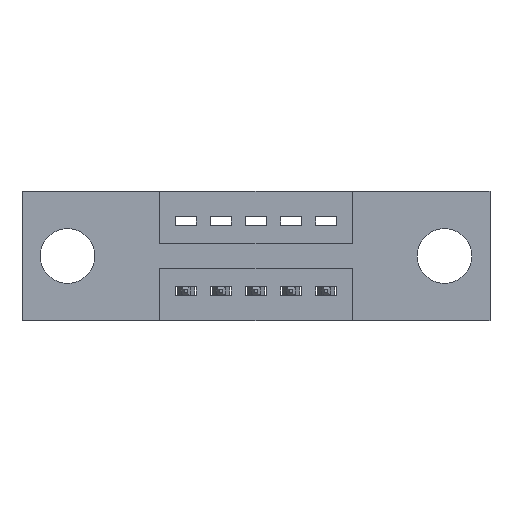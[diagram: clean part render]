
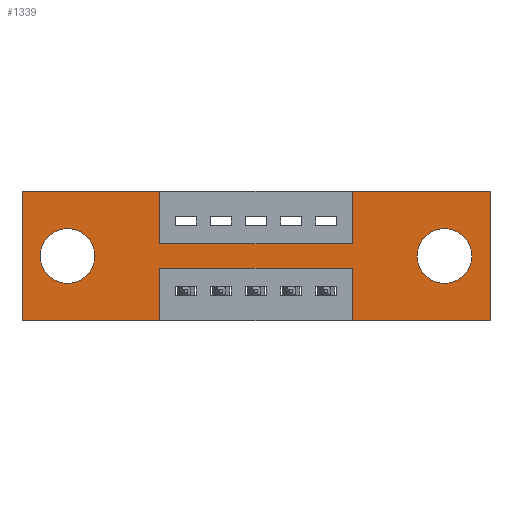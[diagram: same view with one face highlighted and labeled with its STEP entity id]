
A CAD part, front view. The second image highlights one B-rep face of the part: STEP entity #1339.
In plain terms, the highlighted planar face has unit normal (0, -1, 0).
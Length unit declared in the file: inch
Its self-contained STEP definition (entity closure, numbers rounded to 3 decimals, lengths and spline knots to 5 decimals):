
#39 = VECTOR ( 'NONE', #539, 39.37008 ) ;
#45 = VERTEX_POINT ( 'NONE', #7832 ) ;
#56 = VERTEX_POINT ( 'NONE', #8480 ) ;
#64 = CARTESIAN_POINT ( 'NONE',  ( 1.205, 0., -0.263 ) ) ;
#68 = EDGE_CURVE ( 'NONE', #2637, #4759, #3642, .T. ) ;
#254 = CARTESIAN_POINT ( 'NONE',  ( 0.3925, 0., 0. ) ) ;
#285 = LINE ( 'NONE', #3169, #6227 ) ;
#312 = CARTESIAN_POINT ( 'NONE',  ( 0.9425, 0., -0.37 ) ) ;
#321 = ORIENTED_EDGE ( 'NONE', *, *, #921, .F. ) ;
#461 = DIRECTION ( 'NONE',  ( 0., 0., -1. ) ) ;
#539 = DIRECTION ( 'NONE',  ( 0., 0., 1. ) ) ;
#630 = LINE ( 'NONE', #2152, #6124 ) ;
#632 = DIRECTION ( 'NONE',  ( 0., 0., 1. ) ) ;
#645 = VERTEX_POINT ( 'NONE', #5181 ) ;
#648 = LINE ( 'NONE', #6336, #7544 ) ;
#671 = DIRECTION ( 'NONE',  ( 1., 0., 0. ) ) ;
#755 = AXIS2_PLACEMENT_3D ( 'NONE', #7624, #4739, #4033 ) ;
#921 = EDGE_CURVE ( 'NONE', #1124, #2637, #5631, .T. ) ;
#926 = VERTEX_POINT ( 'NONE', #6422 ) ;
#1000 = CIRCLE ( 'NONE', #2480, 0.078 ) ;
#1013 = CARTESIAN_POINT ( 'NONE',  ( 0.13, 0., -0.185 ) ) ;
#1027 = DIRECTION ( 'NONE',  ( 1., 0., 0. ) ) ;
#1090 = EDGE_CURVE ( 'NONE', #9175, #8445, #7405, .T. ) ;
#1119 = VERTEX_POINT ( 'NONE', #8968 ) ;
#1124 = VERTEX_POINT ( 'NONE', #312 ) ;
#1145 = CARTESIAN_POINT ( 'NONE',  ( 0., 0., 0. ) ) ;
#1160 = CARTESIAN_POINT ( 'NONE',  ( 0.3925, 0., -0.22 ) ) ;
#1339 = ADVANCED_FACE ( 'NONE', ( #4218, #2721, #5574 ), #6368, .T. ) ;
#1470 = ORIENTED_EDGE ( 'NONE', *, *, #7257, .F. ) ;
#1474 = DIRECTION ( 'NONE',  ( 0., 1., 0. ) ) ;
#1566 = DIRECTION ( 'NONE',  ( 0., 0., 1. ) ) ;
#1571 = VERTEX_POINT ( 'NONE', #4639 ) ;
#1791 = CARTESIAN_POINT ( 'NONE',  ( 1.335, 0., 0. ) ) ;
#1833 = ORIENTED_EDGE ( 'NONE', *, *, #6652, .T. ) ;
#1836 = DIRECTION ( 'NONE',  ( 1., 0., 0. ) ) ;
#1928 = ORIENTED_EDGE ( 'NONE', *, *, #2625, .F. ) ;
#1961 = ORIENTED_EDGE ( 'NONE', *, *, #68, .F. ) ;
#2019 = DIRECTION ( 'NONE',  ( 0., 0., -1. ) ) ;
#2105 = AXIS2_PLACEMENT_3D ( 'NONE', #6806, #9021, #8374 ) ;
#2146 = CARTESIAN_POINT ( 'NONE',  ( 0.9425, 0., -0.15 ) ) ;
#2152 = CARTESIAN_POINT ( 'NONE',  ( 0.3925, 0., -0.15 ) ) ;
#2214 = EDGE_CURVE ( 'NONE', #645, #1571, #285, .T. ) ;
#2242 = CARTESIAN_POINT ( 'NONE',  ( 0., 0., -0.37 ) ) ;
#2480 = AXIS2_PLACEMENT_3D ( 'NONE', #5217, #1474, #8046 ) ;
#2595 = LINE ( 'NONE', #3302, #3002 ) ;
#2625 = EDGE_CURVE ( 'NONE', #45, #8987, #6097, .T. ) ;
#2637 = VERTEX_POINT ( 'NONE', #6051 ) ;
#2721 = FACE_BOUND ( 'NONE', #3442, .T. ) ;
#2758 = EDGE_CURVE ( 'NONE', #1571, #926, #8178, .T. ) ;
#2879 = VERTEX_POINT ( 'NONE', #64 ) ;
#2892 = DIRECTION ( 'NONE',  ( -1., 0., 0. ) ) ;
#2906 = CARTESIAN_POINT ( 'NONE',  ( 0.9425, 0., 0. ) ) ;
#3002 = VECTOR ( 'NONE', #461, 39.37008 ) ;
#3169 = CARTESIAN_POINT ( 'NONE',  ( 0., 0., 0. ) ) ;
#3302 = CARTESIAN_POINT ( 'NONE',  ( 0.3925, 0., 0. ) ) ;
#3384 = VERTEX_POINT ( 'NONE', #4531 ) ;
#3442 = EDGE_LOOP ( 'NONE', ( #6928, #1833 ) ) ;
#3567 = DIRECTION ( 'NONE',  ( 0., 0., 1. ) ) ;
#3642 = LINE ( 'NONE', #7056, #7524 ) ;
#3647 = EDGE_CURVE ( 'NONE', #1119, #4884, #648, .T. ) ;
#3790 = VECTOR ( 'NONE', #4559, 39.37008 ) ;
#3804 = EDGE_CURVE ( 'NONE', #3384, #2879, #1000, .T. ) ;
#3900 = CARTESIAN_POINT ( 'NONE',  ( 0., 0., 0. ) ) ;
#4033 = DIRECTION ( 'NONE',  ( 0., 0., -1. ) ) ;
#4218 = FACE_BOUND ( 'NONE', #9081, .T. ) ;
#4230 = CARTESIAN_POINT ( 'NONE',  ( 0.9425, 0., -0.37 ) ) ;
#4273 = EDGE_LOOP ( 'NONE', ( #1470, #1961, #321, #4582, #7538, #7606, #7416, #6648, #6866, #1928, #7361, #8955 ) ) ;
#4360 = LINE ( 'NONE', #2906, #7036 ) ;
#4531 = CARTESIAN_POINT ( 'NONE',  ( 1.205, 0., -0.107 ) ) ;
#4559 = DIRECTION ( 'NONE',  ( 0., 0., -1. ) ) ;
#4582 = ORIENTED_EDGE ( 'NONE', *, *, #4722, .F. ) ;
#4589 = CARTESIAN_POINT ( 'NONE',  ( 0.13, 0., -0.107 ) ) ;
#4639 = CARTESIAN_POINT ( 'NONE',  ( 1.335, 0., 0. ) ) ;
#4700 = VERTEX_POINT ( 'NONE', #2146 ) ;
#4722 = EDGE_CURVE ( 'NONE', #926, #1124, #5657, .T. ) ;
#4739 = DIRECTION ( 'NONE',  ( 0., 1., 0. ) ) ;
#4759 = VERTEX_POINT ( 'NONE', #1160 ) ;
#4876 = DIRECTION ( 'NONE',  ( 0., 0., -1. ) ) ;
#4884 = VERTEX_POINT ( 'NONE', #8380 ) ;
#5181 = CARTESIAN_POINT ( 'NONE',  ( 0.9425, 0., 0. ) ) ;
#5217 = CARTESIAN_POINT ( 'NONE',  ( 1.205, 0., -0.185 ) ) ;
#5338 = ORIENTED_EDGE ( 'NONE', *, *, #7166, .T. ) ;
#5397 = CIRCLE ( 'NONE', #755, 0.078 ) ;
#5529 = CARTESIAN_POINT ( 'NONE',  ( 0.3925, 0., -0.37 ) ) ;
#5530 = CARTESIAN_POINT ( 'NONE',  ( 0., 0., -0.37 ) ) ;
#5574 = FACE_OUTER_BOUND ( 'NONE', #4273, .T. ) ;
#5631 = LINE ( 'NONE', #4230, #6203 ) ;
#5657 = LINE ( 'NONE', #2242, #8604 ) ;
#6051 = CARTESIAN_POINT ( 'NONE',  ( 0.9425, 0., -0.22 ) ) ;
#6097 = LINE ( 'NONE', #3900, #7428 ) ;
#6124 = VECTOR ( 'NONE', #671, 39.37008 ) ;
#6152 = ORIENTED_EDGE ( 'NONE', *, *, #3804, .T. ) ;
#6203 = VECTOR ( 'NONE', #3567, 39.37008 ) ;
#6227 = VECTOR ( 'NONE', #1027, 39.37008 ) ;
#6336 = CARTESIAN_POINT ( 'NONE',  ( 0., 0., -0.37 ) ) ;
#6368 = PLANE ( 'NONE',  #9019 ) ;
#6384 = DIRECTION ( 'NONE',  ( -1., 0., 0. ) ) ;
#6417 = VECTOR ( 'NONE', #4876, 39.37008 ) ;
#6422 = CARTESIAN_POINT ( 'NONE',  ( 1.335, 0., -0.37 ) ) ;
#6473 = DIRECTION ( 'NONE',  ( 0., 1., 0. ) ) ;
#6548 = DIRECTION ( 'NONE',  ( -1., 0., 0. ) ) ;
#6635 = EDGE_CURVE ( 'NONE', #8987, #56, #2595, .T. ) ;
#6648 = ORIENTED_EDGE ( 'NONE', *, *, #7287, .F. ) ;
#6652 = EDGE_CURVE ( 'NONE', #8445, #9175, #7032, .T. ) ;
#6806 = CARTESIAN_POINT ( 'NONE',  ( 0.13, 0., -0.185 ) ) ;
#6866 = ORIENTED_EDGE ( 'NONE', *, *, #6635, .F. ) ;
#6928 = ORIENTED_EDGE ( 'NONE', *, *, #1090, .T. ) ;
#7032 = CIRCLE ( 'NONE', #2105, 0.078 ) ;
#7036 = VECTOR ( 'NONE', #632, 39.37008 ) ;
#7056 = CARTESIAN_POINT ( 'NONE',  ( 0.3925, 0., -0.22 ) ) ;
#7166 = EDGE_CURVE ( 'NONE', #2879, #3384, #5397, .T. ) ;
#7257 = EDGE_CURVE ( 'NONE', #4759, #1119, #9098, .T. ) ;
#7262 = AXIS2_PLACEMENT_3D ( 'NONE', #1013, #6473, #1566 ) ;
#7287 = EDGE_CURVE ( 'NONE', #56, #4700, #630, .T. ) ;
#7361 = ORIENTED_EDGE ( 'NONE', *, *, #8361, .F. ) ;
#7405 = CIRCLE ( 'NONE', #7262, 0.078 ) ;
#7416 = ORIENTED_EDGE ( 'NONE', *, *, #8416, .F. ) ;
#7428 = VECTOR ( 'NONE', #1836, 39.37008 ) ;
#7524 = VECTOR ( 'NONE', #2892, 39.37008 ) ;
#7537 = LINE ( 'NONE', #1145, #39 ) ;
#7538 = ORIENTED_EDGE ( 'NONE', *, *, #2758, .F. ) ;
#7544 = VECTOR ( 'NONE', #6384, 39.37008 ) ;
#7606 = ORIENTED_EDGE ( 'NONE', *, *, #2214, .F. ) ;
#7624 = CARTESIAN_POINT ( 'NONE',  ( 1.205, 0., -0.185 ) ) ;
#7832 = CARTESIAN_POINT ( 'NONE',  ( 0., 0., 0. ) ) ;
#8046 = DIRECTION ( 'NONE',  ( 0., 0., -1. ) ) ;
#8178 = LINE ( 'NONE', #1791, #3790 ) ;
#8361 = EDGE_CURVE ( 'NONE', #4884, #45, #7537, .T. ) ;
#8374 = DIRECTION ( 'NONE',  ( 0., 0., 1. ) ) ;
#8380 = CARTESIAN_POINT ( 'NONE',  ( 0., 0., -0.37 ) ) ;
#8405 = DIRECTION ( 'NONE',  ( 0., -1., 0. ) ) ;
#8416 = EDGE_CURVE ( 'NONE', #4700, #645, #4360, .T. ) ;
#8445 = VERTEX_POINT ( 'NONE', #9190 ) ;
#8480 = CARTESIAN_POINT ( 'NONE',  ( 0.3925, 0., -0.15 ) ) ;
#8604 = VECTOR ( 'NONE', #6548, 39.37008 ) ;
#8955 = ORIENTED_EDGE ( 'NONE', *, *, #3647, .F. ) ;
#8968 = CARTESIAN_POINT ( 'NONE',  ( 0.3925, 0., -0.37 ) ) ;
#8987 = VERTEX_POINT ( 'NONE', #254 ) ;
#9019 = AXIS2_PLACEMENT_3D ( 'NONE', #5530, #8405, #2019 ) ;
#9021 = DIRECTION ( 'NONE',  ( 0., 1., 0. ) ) ;
#9081 = EDGE_LOOP ( 'NONE', ( #6152, #5338 ) ) ;
#9098 = LINE ( 'NONE', #5529, #6417 ) ;
#9175 = VERTEX_POINT ( 'NONE', #4589 ) ;
#9190 = CARTESIAN_POINT ( 'NONE',  ( 0.13, 0., -0.263 ) ) ;
